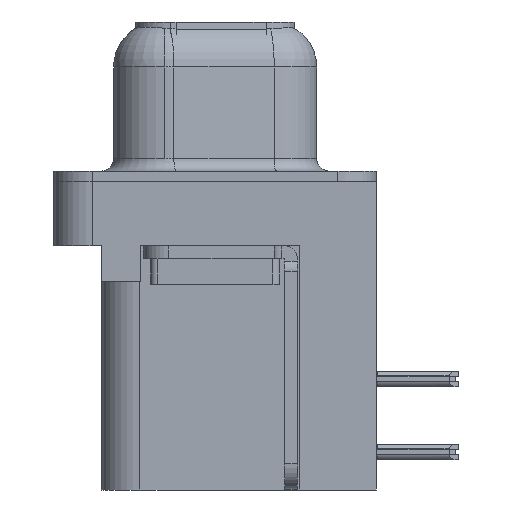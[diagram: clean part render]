
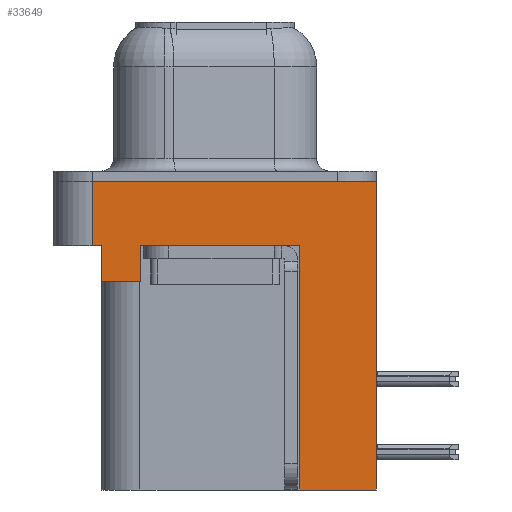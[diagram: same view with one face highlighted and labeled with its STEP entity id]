
A CAD part, left-side view. The second image highlights one B-rep face of the part: STEP entity #33649.
In plain terms, the highlighted planar face has unit normal (-1, 0, 0).
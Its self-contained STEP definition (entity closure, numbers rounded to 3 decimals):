
#94 = VERTEX_POINT ( 'NONE', #34072 ) ;
#472 = ORIENTED_EDGE ( 'NONE', *, *, #3009, .F. ) ;
#483 = DIRECTION ( 'NONE',  ( 0., 1., 0. ) ) ;
#508 = DIRECTION ( 'NONE',  ( 0., 0., 1. ) ) ;
#540 = DIRECTION ( 'NONE',  ( 0., -1., 0. ) ) ;
#627 = CARTESIAN_POINT ( 'NONE',  ( -2.91, 4.775, -2.5 ) ) ;
#654 = DIRECTION ( 'NONE',  ( 0., 0., 1. ) ) ;
#907 = LINE ( 'NONE', #29365, #3821 ) ;
#1004 = VECTOR ( 'NONE', #21695, 1000. ) ;
#1340 = EDGE_CURVE ( 'NONE', #19931, #5928, #21853, .T. ) ;
#1345 = ORIENTED_EDGE ( 'NONE', *, *, #26947, .T. ) ;
#1390 = VERTEX_POINT ( 'NONE', #3356 ) ;
#1606 = DIRECTION ( 'NONE',  ( 0., 0., 1. ) ) ;
#2142 = CARTESIAN_POINT ( 'NONE',  ( -2.91, -6.275, 0. ) ) ;
#2246 = VECTOR ( 'NONE', #21036, 1000. ) ;
#2593 = CARTESIAN_POINT ( 'NONE',  ( -2.91, 4.425, -3.9 ) ) ;
#2970 = VECTOR ( 'NONE', #540, 1000. ) ;
#3009 = EDGE_CURVE ( 'NONE', #9415, #7370, #3092, .T. ) ;
#3092 = LINE ( 'NONE', #627, #1004 ) ;
#3356 = CARTESIAN_POINT ( 'NONE',  ( -2.91, 2.895, -3.9 ) ) ;
#3821 = VECTOR ( 'NONE', #508, 1000. ) ;
#3859 = EDGE_CURVE ( 'NONE', #19931, #94, #17266, .T. ) ;
#3905 = EDGE_CURVE ( 'NONE', #10020, #33875, #21774, .T. ) ;
#3980 = DIRECTION ( 'NONE',  ( 0., 0., 1. ) ) ;
#4018 = VECTOR ( 'NONE', #483, 1000. ) ;
#5563 = VERTEX_POINT ( 'NONE', #27117 ) ;
#5607 = CARTESIAN_POINT ( 'NONE',  ( -2.91, -6.275, 0. ) ) ;
#5928 = VERTEX_POINT ( 'NONE', #2142 ) ;
#6806 = ORIENTED_EDGE ( 'NONE', *, *, #28496, .F. ) ;
#7064 = LINE ( 'NONE', #5607, #12430 ) ;
#7370 = VERTEX_POINT ( 'NONE', #28187 ) ;
#8461 = CARTESIAN_POINT ( 'NONE',  ( -2.91, 4.425, -3.9 ) ) ;
#9415 = VERTEX_POINT ( 'NONE', #32748 ) ;
#10020 = VERTEX_POINT ( 'NONE', #25935 ) ;
#10263 = VECTOR ( 'NONE', #26381, 1000. ) ;
#10693 = VECTOR ( 'NONE', #25636, 1000. ) ;
#10766 = FACE_OUTER_BOUND ( 'NONE', #31576, .T. ) ;
#12430 = VECTOR ( 'NONE', #23994, 1000. ) ;
#13438 = ORIENTED_EDGE ( 'NONE', *, *, #16331, .F. ) ;
#13827 = ORIENTED_EDGE ( 'NONE', *, *, #24978, .T. ) ;
#14051 = ORIENTED_EDGE ( 'NONE', *, *, #18052, .F. ) ;
#14373 = CARTESIAN_POINT ( 'NONE',  ( -2.91, -3.295, -12. ) ) ;
#15691 = CARTESIAN_POINT ( 'NONE',  ( -2.91, 4.425, -2.5 ) ) ;
#16331 = EDGE_CURVE ( 'NONE', #7370, #5928, #7064, .T. ) ;
#16952 = PLANE ( 'NONE',  #28886 ) ;
#17266 = LINE ( 'NONE', #14373, #10693 ) ;
#18052 = EDGE_CURVE ( 'NONE', #1390, #10020, #20868, .T. ) ;
#18095 = VERTEX_POINT ( 'NONE', #21342 ) ;
#19931 = VERTEX_POINT ( 'NONE', #29055 ) ;
#20172 = VECTOR ( 'NONE', #654, 1000. ) ;
#20868 = LINE ( 'NONE', #8461, #4018 ) ;
#21036 = DIRECTION ( 'NONE',  ( 0., -1., 0. ) ) ;
#21342 = CARTESIAN_POINT ( 'NONE',  ( -2.91, -3.295, -2.5 ) ) ;
#21366 = LINE ( 'NONE', #30878, #31631 ) ;
#21695 = DIRECTION ( 'NONE',  ( 0., 0., 1. ) ) ;
#21774 = LINE ( 'NONE', #2593, #10263 ) ;
#21853 = LINE ( 'NONE', #32601, #20172 ) ;
#22271 = LINE ( 'NONE', #31915, #2970 ) ;
#23994 = DIRECTION ( 'NONE',  ( 0., -1., 0. ) ) ;
#24055 = LINE ( 'NONE', #26080, #2246 ) ;
#24978 = EDGE_CURVE ( 'NONE', #9415, #33875, #24055, .T. ) ;
#25636 = DIRECTION ( 'NONE',  ( 0., 1., 0. ) ) ;
#25935 = CARTESIAN_POINT ( 'NONE',  ( -2.91, 4.425, -3.9 ) ) ;
#26080 = CARTESIAN_POINT ( 'NONE',  ( -2.91, -6.275, -2.5 ) ) ;
#26381 = DIRECTION ( 'NONE',  ( 0., 0., 1. ) ) ;
#26947 = EDGE_CURVE ( 'NONE', #5563, #18095, #22271, .T. ) ;
#27117 = CARTESIAN_POINT ( 'NONE',  ( -2.91, 2.895, -2.5 ) ) ;
#27148 = CARTESIAN_POINT ( 'NONE',  ( -2.91, -6.275, -2.5 ) ) ;
#27266 = DIRECTION ( 'NONE',  ( -1., 0., 0. ) ) ;
#27349 = ORIENTED_EDGE ( 'NONE', *, *, #1340, .T. ) ;
#28187 = CARTESIAN_POINT ( 'NONE',  ( -2.91, 4.775, 0. ) ) ;
#28496 = EDGE_CURVE ( 'NONE', #94, #18095, #21366, .T. ) ;
#28733 = ORIENTED_EDGE ( 'NONE', *, *, #3859, .F. ) ;
#28886 = AXIS2_PLACEMENT_3D ( 'NONE', #27148, #27266, #3980 ) ;
#29055 = CARTESIAN_POINT ( 'NONE',  ( -2.91, -6.275, -12. ) ) ;
#29365 = CARTESIAN_POINT ( 'NONE',  ( -2.91, 2.895, -3.9 ) ) ;
#30878 = CARTESIAN_POINT ( 'NONE',  ( -2.91, -3.295, -12. ) ) ;
#31576 = EDGE_LOOP ( 'NONE', ( #13438, #472, #13827, #32811, #14051, #33334, #1345, #6806, #28733, #27349 ) ) ;
#31631 = VECTOR ( 'NONE', #1606, 1000. ) ;
#31915 = CARTESIAN_POINT ( 'NONE',  ( -2.91, -6.275, -2.5 ) ) ;
#32601 = CARTESIAN_POINT ( 'NONE',  ( -2.91, -6.275, -2.5 ) ) ;
#32748 = CARTESIAN_POINT ( 'NONE',  ( -2.91, 4.775, -2.5 ) ) ;
#32811 = ORIENTED_EDGE ( 'NONE', *, *, #3905, .F. ) ;
#32936 = EDGE_CURVE ( 'NONE', #1390, #5563, #907, .T. ) ;
#33334 = ORIENTED_EDGE ( 'NONE', *, *, #32936, .T. ) ;
#33649 = ADVANCED_FACE ( 'NONE', ( #10766 ), #16952, .T. ) ;
#33875 = VERTEX_POINT ( 'NONE', #15691 ) ;
#34072 = CARTESIAN_POINT ( 'NONE',  ( -2.91, -3.295, -12. ) ) ;
